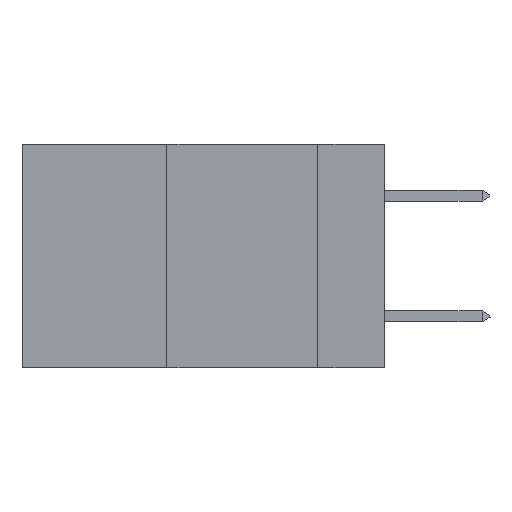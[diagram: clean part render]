
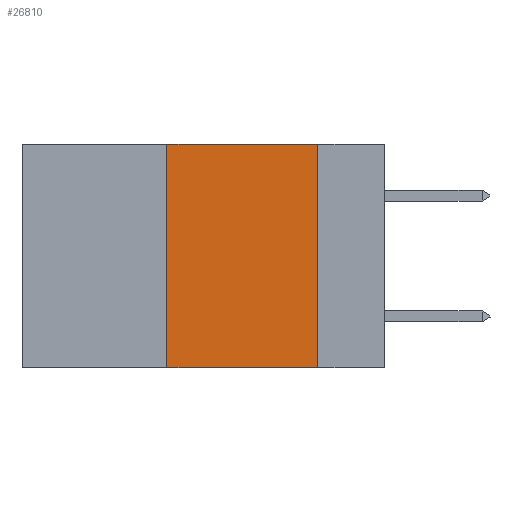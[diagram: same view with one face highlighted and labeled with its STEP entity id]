
A CAD part, left-side view. The second image highlights one B-rep face of the part: STEP entity #26810.
In plain terms, the highlighted planar face has unit normal (-1, 0, 0).
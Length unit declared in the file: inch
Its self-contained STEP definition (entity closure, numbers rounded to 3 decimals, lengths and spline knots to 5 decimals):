
#169 = LINE ( 'NONE', #5097, #12255 ) ;
#430 = VERTEX_POINT ( 'NONE', #10854 ) ;
#807 = EDGE_CURVE ( 'NONE', #430, #25875, #2443, .T. ) ;
#2241 = FACE_OUTER_BOUND ( 'NONE', #15191, .T. ) ;
#2443 = LINE ( 'NONE', #26750, #19827 ) ;
#2568 = DIRECTION ( 'NONE',  ( 0., 0., -1. ) ) ;
#5097 = CARTESIAN_POINT ( 'NONE',  ( 0., 0.6, 0. ) ) ;
#5118 = ORIENTED_EDGE ( 'NONE', *, *, #30196, .T. ) ;
#6202 = CARTESIAN_POINT ( 'NONE',  ( 0., 0.36, 0. ) ) ;
#10103 = DIRECTION ( 'NONE',  ( 1., 0., 0. ) ) ;
#10854 = CARTESIAN_POINT ( 'NONE',  ( 0., 0.11, 0. ) ) ;
#12255 = VECTOR ( 'NONE', #26965, 39.37008 ) ;
#12414 = CARTESIAN_POINT ( 'NONE',  ( 0., 0.36, -0.37 ) ) ;
#12798 = EDGE_CURVE ( 'NONE', #20718, #17885, #24921, .T. ) ;
#15066 = DIRECTION ( 'NONE',  ( 0., 0., -1. ) ) ;
#15191 = EDGE_LOOP ( 'NONE', ( #21988, #30931, #15781, #5118 ) ) ;
#15781 = ORIENTED_EDGE ( 'NONE', *, *, #12798, .F. ) ;
#15953 = CARTESIAN_POINT ( 'NONE',  ( 0., 0.6, -0.37 ) ) ;
#16568 = AXIS2_PLACEMENT_3D ( 'NONE', #27013, #10103, #15066 ) ;
#17885 = VERTEX_POINT ( 'NONE', #6202 ) ;
#18273 = DIRECTION ( 'NONE',  ( 0., -1., 0. ) ) ;
#18669 = VECTOR ( 'NONE', #18273, 39.37008 ) ;
#19827 = VECTOR ( 'NONE', #2568, 39.37008 ) ;
#20718 = VERTEX_POINT ( 'NONE', #12414 ) ;
#21988 = ORIENTED_EDGE ( 'NONE', *, *, #807, .F. ) ;
#23081 = EDGE_CURVE ( 'NONE', #17885, #430, #169, .T. ) ;
#23162 = CARTESIAN_POINT ( 'NONE',  ( 0., 0.36, 0. ) ) ;
#24177 = PLANE ( 'NONE',  #16568 ) ;
#24707 = LINE ( 'NONE', #15953, #18669 ) ;
#24921 = LINE ( 'NONE', #23162, #30615 ) ;
#25123 = CARTESIAN_POINT ( 'NONE',  ( 0., 0.11, -0.37 ) ) ;
#25875 = VERTEX_POINT ( 'NONE', #25123 ) ;
#26750 = CARTESIAN_POINT ( 'NONE',  ( 0., 0.11, 0. ) ) ;
#26810 = ADVANCED_FACE ( 'NONE', ( #2241 ), #24177, .F. ) ;
#26965 = DIRECTION ( 'NONE',  ( 0., -1., 0. ) ) ;
#27013 = CARTESIAN_POINT ( 'NONE',  ( 0., 0.6, 0. ) ) ;
#28128 = DIRECTION ( 'NONE',  ( 0., 0., 1. ) ) ;
#30196 = EDGE_CURVE ( 'NONE', #20718, #25875, #24707, .T. ) ;
#30615 = VECTOR ( 'NONE', #28128, 39.37008 ) ;
#30931 = ORIENTED_EDGE ( 'NONE', *, *, #23081, .F. ) ;
